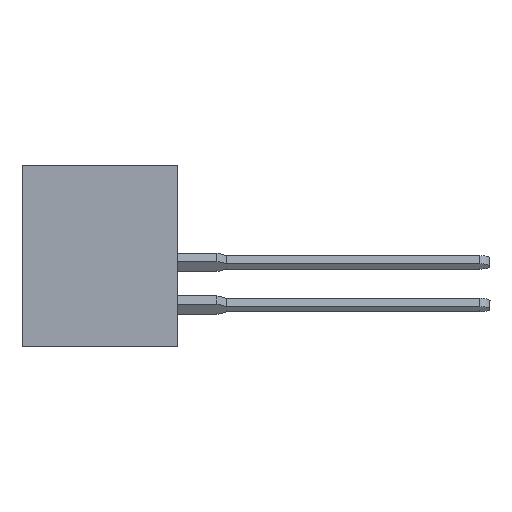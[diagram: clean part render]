
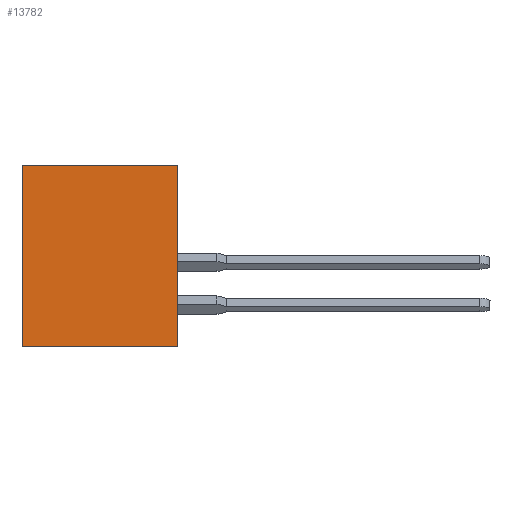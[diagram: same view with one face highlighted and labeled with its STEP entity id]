
A CAD part, left-side view. The second image highlights one B-rep face of the part: STEP entity #13782.
In plain terms, the highlighted planar face has unit normal (-1, 0, 0).
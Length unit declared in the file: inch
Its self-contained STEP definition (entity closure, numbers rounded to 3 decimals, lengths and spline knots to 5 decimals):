
#608 = VECTOR ( 'NONE', #17693, 39.37008 ) ;
#640 = CARTESIAN_POINT ( 'NONE',  ( 0., 0., -0.531 ) ) ;
#1071 = EDGE_CURVE ( 'NONE', #19912, #26085, #15355, .T. ) ;
#1139 = DIRECTION ( 'NONE',  ( 0., 0., 1. ) ) ;
#1379 = CARTESIAN_POINT ( 'NONE',  ( 0., 0.453, 0. ) ) ;
#1554 = EDGE_CURVE ( 'NONE', #7461, #7118, #23309, .T. ) ;
#2189 = CARTESIAN_POINT ( 'NONE',  ( 0., 0., 0. ) ) ;
#3203 = CARTESIAN_POINT ( 'NONE',  ( 0., 0.453, -0.531 ) ) ;
#5274 = EDGE_CURVE ( 'NONE', #26085, #7118, #22115, .T. ) ;
#6779 = DIRECTION ( 'NONE',  ( 1., 0., 0. ) ) ;
#6785 = DIRECTION ( 'NONE',  ( 0., -1., 0. ) ) ;
#7118 = VERTEX_POINT ( 'NONE', #14415 ) ;
#7461 = VERTEX_POINT ( 'NONE', #640 ) ;
#9536 = ORIENTED_EDGE ( 'NONE', *, *, #1554, .T. ) ;
#11796 = FACE_OUTER_BOUND ( 'NONE', #27369, .T. ) ;
#12216 = ORIENTED_EDGE ( 'NONE', *, *, #25299, .T. ) ;
#13489 = DIRECTION ( 'NONE',  ( 0., 0., -1. ) ) ;
#13782 = ADVANCED_FACE ( 'NONE', ( #11796 ), #26219, .F. ) ;
#14415 = CARTESIAN_POINT ( 'NONE',  ( 0., 0., 0. ) ) ;
#15068 = DIRECTION ( 'NONE',  ( 0., 0., 1. ) ) ;
#15355 = LINE ( 'NONE', #26153, #20341 ) ;
#17493 = CARTESIAN_POINT ( 'NONE',  ( 0., 0.453, 0. ) ) ;
#17693 = DIRECTION ( 'NONE',  ( 0., -1., 0. ) ) ;
#19350 = VECTOR ( 'NONE', #6785, 39.37008 ) ;
#19912 = VERTEX_POINT ( 'NONE', #3203 ) ;
#20115 = CARTESIAN_POINT ( 'NONE',  ( 0., 0.453, 0. ) ) ;
#20341 = VECTOR ( 'NONE', #1139, 39.37008 ) ;
#21694 = AXIS2_PLACEMENT_3D ( 'NONE', #17493, #6779, #13489 ) ;
#22115 = LINE ( 'NONE', #20115, #608 ) ;
#22620 = VECTOR ( 'NONE', #15068, 39.37008 ) ;
#23309 = LINE ( 'NONE', #2189, #22620 ) ;
#23991 = CARTESIAN_POINT ( 'NONE',  ( 0., 0.453, -0.531 ) ) ;
#24673 = LINE ( 'NONE', #23991, #19350 ) ;
#25299 = EDGE_CURVE ( 'NONE', #19912, #7461, #24673, .T. ) ;
#25751 = ORIENTED_EDGE ( 'NONE', *, *, #5274, .F. ) ;
#25781 = ORIENTED_EDGE ( 'NONE', *, *, #1071, .F. ) ;
#26085 = VERTEX_POINT ( 'NONE', #1379 ) ;
#26153 = CARTESIAN_POINT ( 'NONE',  ( 0., 0.453, 0. ) ) ;
#26219 = PLANE ( 'NONE',  #21694 ) ;
#27369 = EDGE_LOOP ( 'NONE', ( #9536, #25751, #25781, #12216 ) ) ;
